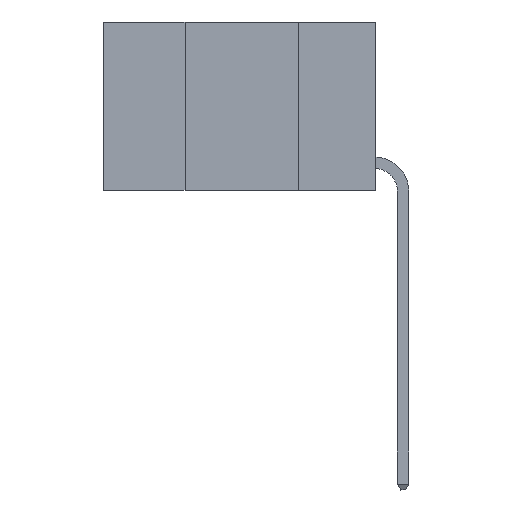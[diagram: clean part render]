
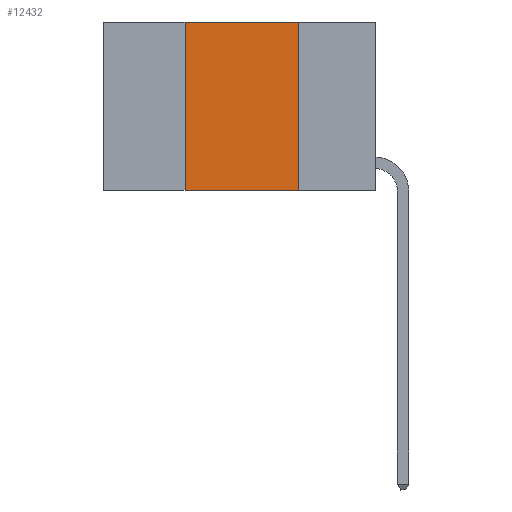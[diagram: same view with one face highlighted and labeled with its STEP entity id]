
A CAD part, left-side view. The second image highlights one B-rep face of the part: STEP entity #12432.
In plain terms, the highlighted planar face has unit normal (-1, 0, 0).
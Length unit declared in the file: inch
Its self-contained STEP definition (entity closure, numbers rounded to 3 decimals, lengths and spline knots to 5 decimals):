
#311 = ORIENTED_EDGE ( 'NONE', *, *, #14955, .F. ) ;
#1437 = ORIENTED_EDGE ( 'NONE', *, *, #8716, .T. ) ;
#1628 = VECTOR ( 'NONE', #7762, 39.37008 ) ;
#1830 = DIRECTION ( 'NONE',  ( 0., -1., 0. ) ) ;
#2485 = ORIENTED_EDGE ( 'NONE', *, *, #3038, .F. ) ;
#3038 = EDGE_CURVE ( 'NONE', #13663, #11881, #16019, .T. ) ;
#3306 = CARTESIAN_POINT ( 'NONE',  ( 0., 0.6, -0.37 ) ) ;
#3591 = VERTEX_POINT ( 'NONE', #3850 ) ;
#3850 = CARTESIAN_POINT ( 'NONE',  ( 0., 0.17, -0.37 ) ) ;
#5341 = PLANE ( 'NONE',  #15277 ) ;
#6039 = DIRECTION ( 'NONE',  ( 0., 0., -1. ) ) ;
#6482 = ORIENTED_EDGE ( 'NONE', *, *, #16343, .F. ) ;
#6484 = LINE ( 'NONE', #17295, #15392 ) ;
#6569 = CARTESIAN_POINT ( 'NONE',  ( 0., 0.17, 0. ) ) ;
#7227 = CARTESIAN_POINT ( 'NONE',  ( 0., 0.42, -0.37 ) ) ;
#7662 = DIRECTION ( 'NONE',  ( 0., 0., 1. ) ) ;
#7762 = DIRECTION ( 'NONE',  ( 0., -1., 0. ) ) ;
#7930 = LINE ( 'NONE', #6569, #14828 ) ;
#7955 = CARTESIAN_POINT ( 'NONE',  ( 0., 0.6, 0. ) ) ;
#8416 = CARTESIAN_POINT ( 'NONE',  ( 0., 0.42, 0. ) ) ;
#8716 = EDGE_CURVE ( 'NONE', #17457, #3591, #10276, .T. ) ;
#9522 = CARTESIAN_POINT ( 'NONE',  ( 0., 0.6, 0. ) ) ;
#9717 = CARTESIAN_POINT ( 'NONE',  ( 0., 0.17, 0. ) ) ;
#10276 = LINE ( 'NONE', #3306, #17405 ) ;
#11881 = VERTEX_POINT ( 'NONE', #9717 ) ;
#12432 = ADVANCED_FACE ( 'NONE', ( #17788 ), #5341, .F. ) ;
#13282 = DIRECTION ( 'NONE',  ( 0., 0., -1. ) ) ;
#13663 = VERTEX_POINT ( 'NONE', #8416 ) ;
#14755 = EDGE_LOOP ( 'NONE', ( #311, #2485, #6482, #1437 ) ) ;
#14828 = VECTOR ( 'NONE', #13282, 39.37008 ) ;
#14955 = EDGE_CURVE ( 'NONE', #11881, #3591, #7930, .T. ) ;
#15052 = DIRECTION ( 'NONE',  ( 1., 0., 0. ) ) ;
#15277 = AXIS2_PLACEMENT_3D ( 'NONE', #9522, #15052, #6039 ) ;
#15392 = VECTOR ( 'NONE', #7662, 39.37008 ) ;
#16019 = LINE ( 'NONE', #7955, #1628 ) ;
#16343 = EDGE_CURVE ( 'NONE', #17457, #13663, #6484, .T. ) ;
#17295 = CARTESIAN_POINT ( 'NONE',  ( 0., 0.42, 0. ) ) ;
#17405 = VECTOR ( 'NONE', #1830, 39.37008 ) ;
#17457 = VERTEX_POINT ( 'NONE', #7227 ) ;
#17788 = FACE_OUTER_BOUND ( 'NONE', #14755, .T. ) ;
